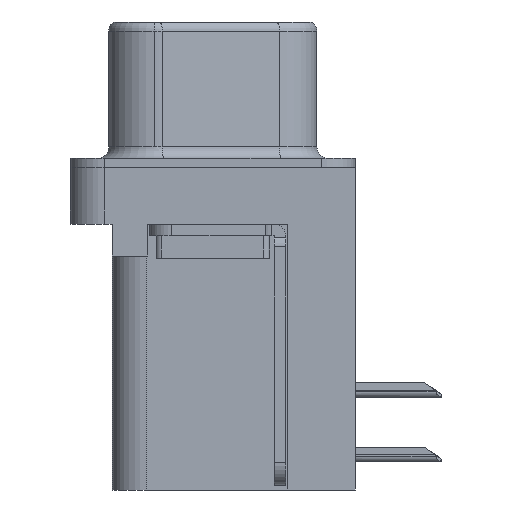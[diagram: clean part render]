
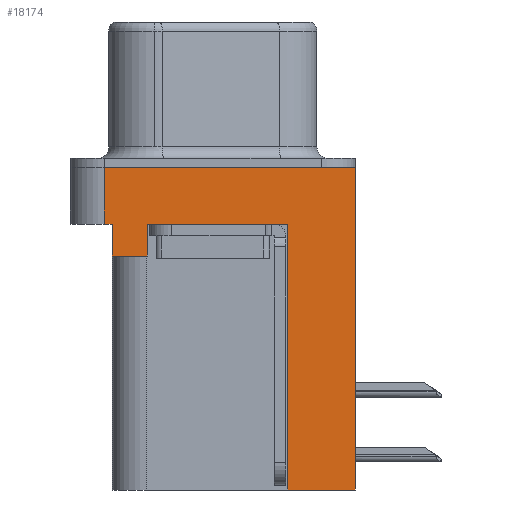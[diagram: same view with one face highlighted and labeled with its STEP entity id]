
A CAD part, left-side view. The second image highlights one B-rep face of the part: STEP entity #18174.
In plain terms, the highlighted planar face has unit normal (-1, 0, 0).
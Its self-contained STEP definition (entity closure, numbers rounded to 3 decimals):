
#904 = ORIENTED_EDGE ( 'NONE', *, *, #5463, .F. ) ;
#1218 = LINE ( 'NONE', #21664, #22612 ) ;
#1307 = LINE ( 'NONE', #21761, #3291 ) ;
#1777 = VECTOR ( 'NONE', #18353, 1000. ) ;
#2071 = EDGE_CURVE ( 'NONE', #20096, #23155, #9317, .T. ) ;
#2150 = DIRECTION ( 'NONE',  ( -1., 0., 0. ) ) ;
#2226 = EDGE_CURVE ( 'NONE', #19139, #11685, #19333, .T. ) ;
#3291 = VECTOR ( 'NONE', #8647, 1000. ) ;
#3370 = CARTESIAN_POINT ( 'NONE',  ( -2.91, 4.425, -3.9 ) ) ;
#3498 = VERTEX_POINT ( 'NONE', #19509 ) ;
#3749 = VERTEX_POINT ( 'NONE', #18504 ) ;
#4444 = VECTOR ( 'NONE', #8122, 1000. ) ;
#4679 = ORIENTED_EDGE ( 'NONE', *, *, #16339, .F. ) ;
#4870 = ORIENTED_EDGE ( 'NONE', *, *, #2071, .T. ) ;
#5187 = DIRECTION ( 'NONE',  ( 0., 1., 0. ) ) ;
#5316 = CARTESIAN_POINT ( 'NONE',  ( -2.91, -6.275, -2.5 ) ) ;
#5463 = EDGE_CURVE ( 'NONE', #15420, #23155, #24060, .T. ) ;
#5840 = CARTESIAN_POINT ( 'NONE',  ( -2.91, -6.275, -2.5 ) ) ;
#6196 = DIRECTION ( 'NONE',  ( 0., -1., 0. ) ) ;
#6374 = VERTEX_POINT ( 'NONE', #23519 ) ;
#6914 = ORIENTED_EDGE ( 'NONE', *, *, #16924, .T. ) ;
#7893 = CARTESIAN_POINT ( 'NONE',  ( -2.91, 4.775, -2.5 ) ) ;
#8122 = DIRECTION ( 'NONE',  ( 0., 0., 1. ) ) ;
#8158 = ORIENTED_EDGE ( 'NONE', *, *, #17329, .F. ) ;
#8300 = CARTESIAN_POINT ( 'NONE',  ( -2.91, -3.295, -2.5 ) ) ;
#8647 = DIRECTION ( 'NONE',  ( 0., 1., 0. ) ) ;
#8670 = LINE ( 'NONE', #16209, #22125 ) ;
#8808 = LINE ( 'NONE', #5316, #21084 ) ;
#8943 = CARTESIAN_POINT ( 'NONE',  ( -2.91, -3.295, -14.2 ) ) ;
#9317 = LINE ( 'NONE', #5840, #13387 ) ;
#9682 = AXIS2_PLACEMENT_3D ( 'NONE', #23331, #2150, #17515 ) ;
#10293 = ORIENTED_EDGE ( 'NONE', *, *, #15613, .F. ) ;
#10867 = DIRECTION ( 'NONE',  ( 0., 0., 1. ) ) ;
#11378 = VECTOR ( 'NONE', #10867, 1000. ) ;
#11537 = VERTEX_POINT ( 'NONE', #19562 ) ;
#11685 = VERTEX_POINT ( 'NONE', #20533 ) ;
#11817 = PLANE ( 'NONE',  #9682 ) ;
#12249 = CARTESIAN_POINT ( 'NONE',  ( -2.91, 2.895, -2.5 ) ) ;
#12868 = DIRECTION ( 'NONE',  ( 0., 0., 1. ) ) ;
#13282 = DIRECTION ( 'NONE',  ( 0., -1., 0. ) ) ;
#13387 = VECTOR ( 'NONE', #13282, 1000. ) ;
#13804 = DIRECTION ( 'NONE',  ( 0., 0., 1. ) ) ;
#13966 = ORIENTED_EDGE ( 'NONE', *, *, #20224, .T. ) ;
#14329 = CARTESIAN_POINT ( 'NONE',  ( -2.91, 4.775, 0. ) ) ;
#14393 = ORIENTED_EDGE ( 'NONE', *, *, #23187, .T. ) ;
#14511 = CARTESIAN_POINT ( 'NONE',  ( -2.91, -3.295, -14.2 ) ) ;
#15420 = VERTEX_POINT ( 'NONE', #14511 ) ;
#15602 = DIRECTION ( 'NONE',  ( 0., -1., 0. ) ) ;
#15613 = EDGE_CURVE ( 'NONE', #6374, #15420, #1218, .T. ) ;
#16209 = CARTESIAN_POINT ( 'NONE',  ( -2.91, -6.275, -2.5 ) ) ;
#16339 = EDGE_CURVE ( 'NONE', #11537, #19139, #19397, .T. ) ;
#16924 = EDGE_CURVE ( 'NONE', #6374, #11685, #8808, .T. ) ;
#17329 = EDGE_CURVE ( 'NONE', #3498, #24357, #1307, .T. ) ;
#17345 = VECTOR ( 'NONE', #15602, 1000. ) ;
#17391 = FACE_OUTER_BOUND ( 'NONE', #21141, .T. ) ;
#17476 = CARTESIAN_POINT ( 'NONE',  ( -2.91, -6.275, 0. ) ) ;
#17515 = DIRECTION ( 'NONE',  ( 0., 0., 1. ) ) ;
#18174 = ADVANCED_FACE ( 'NONE', ( #17391 ), #11817, .T. ) ;
#18353 = DIRECTION ( 'NONE',  ( 0., 0., 1. ) ) ;
#18504 = CARTESIAN_POINT ( 'NONE',  ( -2.91, 4.425, -2.5 ) ) ;
#19130 = CARTESIAN_POINT ( 'NONE',  ( -2.91, 4.425, -3.9 ) ) ;
#19139 = VERTEX_POINT ( 'NONE', #14329 ) ;
#19333 = LINE ( 'NONE', #17476, #17345 ) ;
#19397 = LINE ( 'NONE', #7893, #4444 ) ;
#19500 = EDGE_CURVE ( 'NONE', #24357, #3749, #21467, .T. ) ;
#19509 = CARTESIAN_POINT ( 'NONE',  ( -2.91, 2.895, -3.9 ) ) ;
#19562 = CARTESIAN_POINT ( 'NONE',  ( -2.91, 4.775, -2.5 ) ) ;
#20042 = VECTOR ( 'NONE', #13804, 1000. ) ;
#20096 = VERTEX_POINT ( 'NONE', #12249 ) ;
#20224 = EDGE_CURVE ( 'NONE', #3498, #20096, #22271, .T. ) ;
#20533 = CARTESIAN_POINT ( 'NONE',  ( -2.91, -6.275, 0. ) ) ;
#21084 = VECTOR ( 'NONE', #12868, 1000. ) ;
#21141 = EDGE_LOOP ( 'NONE', ( #24383, #4679, #14393, #21167, #8158, #13966, #4870, #904, #10293, #6914 ) ) ;
#21167 = ORIENTED_EDGE ( 'NONE', *, *, #19500, .F. ) ;
#21467 = LINE ( 'NONE', #19130, #20042 ) ;
#21664 = CARTESIAN_POINT ( 'NONE',  ( -2.91, -3.295, -14.2 ) ) ;
#21761 = CARTESIAN_POINT ( 'NONE',  ( -2.91, 4.425, -3.9 ) ) ;
#22125 = VECTOR ( 'NONE', #6196, 1000. ) ;
#22147 = CARTESIAN_POINT ( 'NONE',  ( -2.91, 2.895, -3.9 ) ) ;
#22271 = LINE ( 'NONE', #22147, #11378 ) ;
#22612 = VECTOR ( 'NONE', #5187, 1000. ) ;
#23155 = VERTEX_POINT ( 'NONE', #8300 ) ;
#23187 = EDGE_CURVE ( 'NONE', #11537, #3749, #8670, .T. ) ;
#23331 = CARTESIAN_POINT ( 'NONE',  ( -2.91, -6.275, -2.5 ) ) ;
#23519 = CARTESIAN_POINT ( 'NONE',  ( -2.91, -6.275, -14.2 ) ) ;
#24060 = LINE ( 'NONE', #8943, #1777 ) ;
#24357 = VERTEX_POINT ( 'NONE', #3370 ) ;
#24383 = ORIENTED_EDGE ( 'NONE', *, *, #2226, .F. ) ;
